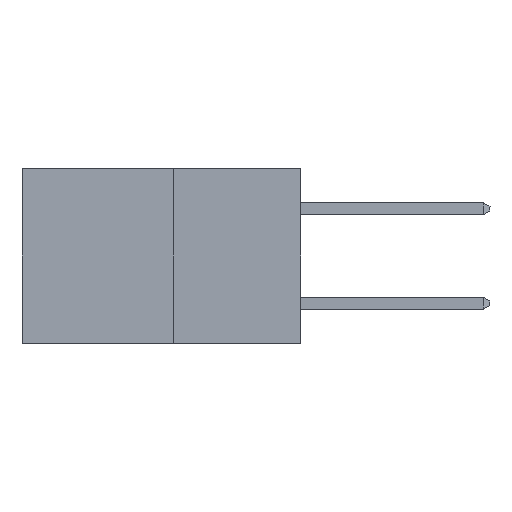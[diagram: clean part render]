
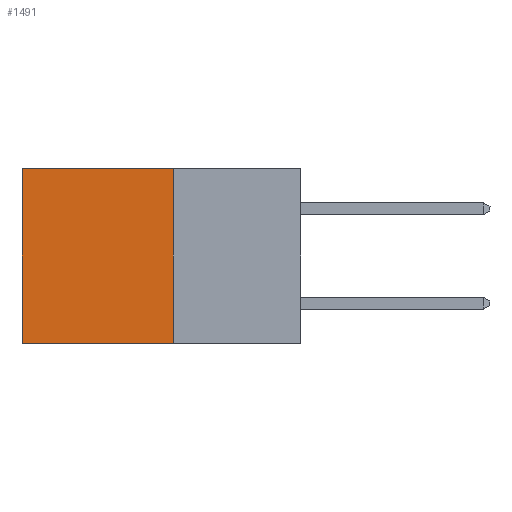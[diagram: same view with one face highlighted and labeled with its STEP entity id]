
A CAD part, left-side view. The second image highlights one B-rep face of the part: STEP entity #1491.
In plain terms, the highlighted planar face has unit normal (-1, 0, 0).
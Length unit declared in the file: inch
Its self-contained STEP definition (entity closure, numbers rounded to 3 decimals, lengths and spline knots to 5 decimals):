
#276 = EDGE_CURVE ( 'NONE', #4011, #1973, #9494, .T. ) ;
#298 = PLANE ( 'NONE',  #877 ) ;
#610 = VECTOR ( 'NONE', #1135, 39.37008 ) ;
#877 = AXIS2_PLACEMENT_3D ( 'NONE', #3637, #3611, #3570 ) ;
#1039 = CARTESIAN_POINT ( 'NONE',  ( 0.277, 0.27, 0. ) ) ;
#1135 = DIRECTION ( 'NONE',  ( 0., 1., 0. ) ) ;
#1462 = DIRECTION ( 'NONE',  ( 0., 1., 0. ) ) ;
#1491 = ADVANCED_FACE ( 'NONE', ( #11195 ), #298, .F. ) ;
#1584 = CARTESIAN_POINT ( 'NONE',  ( 0.277, 0.27, -0.37 ) ) ;
#1633 = LINE ( 'NONE', #1584, #13035 ) ;
#1973 = VERTEX_POINT ( 'NONE', #9712 ) ;
#2504 = ORIENTED_EDGE ( 'NONE', *, *, #7024, .F. ) ;
#2619 = VECTOR ( 'NONE', #8126, 39.37008 ) ;
#3323 = EDGE_CURVE ( 'NONE', #1973, #8783, #14031, .T. ) ;
#3368 = LINE ( 'NONE', #8206, #2619 ) ;
#3570 = DIRECTION ( 'NONE',  ( 0., 0., -1. ) ) ;
#3611 = DIRECTION ( 'NONE',  ( 1., 0., 0. ) ) ;
#3637 = CARTESIAN_POINT ( 'NONE',  ( 0.277, 0.27, -0.37 ) ) ;
#4011 = VERTEX_POINT ( 'NONE', #12333 ) ;
#5088 = VECTOR ( 'NONE', #5831, 39.37008 ) ;
#5134 = CARTESIAN_POINT ( 'NONE',  ( 0.277, 0.59, -0.37 ) ) ;
#5204 = ORIENTED_EDGE ( 'NONE', *, *, #10766, .F. ) ;
#5831 = DIRECTION ( 'NONE',  ( 0., 0., -1. ) ) ;
#5844 = CARTESIAN_POINT ( 'NONE',  ( 0.277, 0.59, -0.37 ) ) ;
#7024 = EDGE_CURVE ( 'NONE', #4011, #14363, #3368, .T. ) ;
#7865 = ORIENTED_EDGE ( 'NONE', *, *, #276, .T. ) ;
#8126 = DIRECTION ( 'NONE',  ( 0., 0., -1. ) ) ;
#8206 = CARTESIAN_POINT ( 'NONE',  ( 0.277, 0.27, -0.37 ) ) ;
#8783 = VERTEX_POINT ( 'NONE', #5134 ) ;
#9494 = LINE ( 'NONE', #1039, #610 ) ;
#9712 = CARTESIAN_POINT ( 'NONE',  ( 0.277, 0.59, 0. ) ) ;
#10766 = EDGE_CURVE ( 'NONE', #14363, #8783, #1633, .T. ) ;
#11195 = FACE_OUTER_BOUND ( 'NONE', #12735, .T. ) ;
#11833 = ORIENTED_EDGE ( 'NONE', *, *, #3323, .T. ) ;
#12333 = CARTESIAN_POINT ( 'NONE',  ( 0.277, 0.27, 0. ) ) ;
#12735 = EDGE_LOOP ( 'NONE', ( #11833, #5204, #2504, #7865 ) ) ;
#13035 = VECTOR ( 'NONE', #1462, 39.37008 ) ;
#14031 = LINE ( 'NONE', #5844, #5088 ) ;
#14363 = VERTEX_POINT ( 'NONE', #14646 ) ;
#14646 = CARTESIAN_POINT ( 'NONE',  ( 0.277, 0.27, -0.37 ) ) ;
